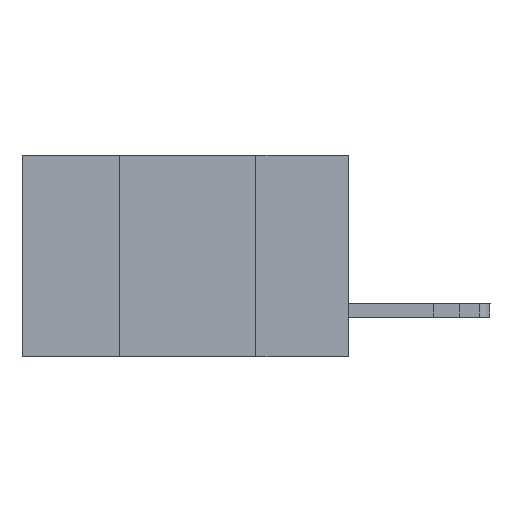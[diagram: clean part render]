
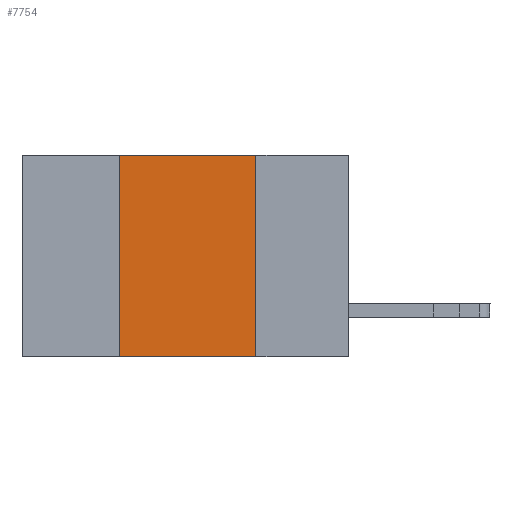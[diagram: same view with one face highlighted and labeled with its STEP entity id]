
A CAD part, left-side view. The second image highlights one B-rep face of the part: STEP entity #7754.
In plain terms, the highlighted planar face has unit normal (-1, 0, 0).
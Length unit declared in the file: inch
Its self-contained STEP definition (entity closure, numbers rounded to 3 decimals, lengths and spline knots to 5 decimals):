
#134 = ORIENTED_EDGE ( 'NONE', *, *, #7679, .F. ) ;
#285 = CARTESIAN_POINT ( 'NONE',  ( 0., 0.6, -0.37 ) ) ;
#486 = VECTOR ( 'NONE', #734, 39.37008 ) ;
#564 = CARTESIAN_POINT ( 'NONE',  ( 0., 0.42, 0. ) ) ;
#578 = VERTEX_POINT ( 'NONE', #10314 ) ;
#629 = CARTESIAN_POINT ( 'NONE',  ( 0., 0.42, -0.37 ) ) ;
#669 = CARTESIAN_POINT ( 'NONE',  ( 0., 0.6, 0. ) ) ;
#734 = DIRECTION ( 'NONE',  ( 0., 0., 1. ) ) ;
#1338 = DIRECTION ( 'NONE',  ( 0., -1., 0. ) ) ;
#1389 = VECTOR ( 'NONE', #5012, 39.37008 ) ;
#1519 = LINE ( 'NONE', #564, #486 ) ;
#1689 = EDGE_CURVE ( 'NONE', #7412, #578, #9276, .T. ) ;
#1795 = DIRECTION ( 'NONE',  ( 1., 0., 0. ) ) ;
#2260 = EDGE_LOOP ( 'NONE', ( #8542, #10179, #134, #9044 ) ) ;
#2490 = VERTEX_POINT ( 'NONE', #629 ) ;
#2897 = DIRECTION ( 'NONE',  ( 0., 0., -1. ) ) ;
#3389 = VECTOR ( 'NONE', #2897, 39.37008 ) ;
#3930 = VECTOR ( 'NONE', #1338, 39.37008 ) ;
#4408 = DIRECTION ( 'NONE',  ( 0., 0., -1. ) ) ;
#5012 = DIRECTION ( 'NONE',  ( 0., -1., 0. ) ) ;
#7232 = CARTESIAN_POINT ( 'NONE',  ( 0., 0.17, 0. ) ) ;
#7412 = VERTEX_POINT ( 'NONE', #10342 ) ;
#7679 = EDGE_CURVE ( 'NONE', #2490, #7412, #1519, .T. ) ;
#7754 = ADVANCED_FACE ( 'NONE', ( #9344 ), #8678, .F. ) ;
#8469 = VERTEX_POINT ( 'NONE', #9132 ) ;
#8542 = ORIENTED_EDGE ( 'NONE', *, *, #9476, .F. ) ;
#8678 = PLANE ( 'NONE',  #9589 ) ;
#9044 = ORIENTED_EDGE ( 'NONE', *, *, #9055, .T. ) ;
#9055 = EDGE_CURVE ( 'NONE', #2490, #8469, #10663, .T. ) ;
#9132 = CARTESIAN_POINT ( 'NONE',  ( 0., 0.17, -0.37 ) ) ;
#9276 = LINE ( 'NONE', #669, #1389 ) ;
#9344 = FACE_OUTER_BOUND ( 'NONE', #2260, .T. ) ;
#9397 = CARTESIAN_POINT ( 'NONE',  ( 0., 0.6, 0. ) ) ;
#9476 = EDGE_CURVE ( 'NONE', #578, #8469, #9601, .T. ) ;
#9589 = AXIS2_PLACEMENT_3D ( 'NONE', #9397, #1795, #4408 ) ;
#9601 = LINE ( 'NONE', #7232, #3389 ) ;
#10179 = ORIENTED_EDGE ( 'NONE', *, *, #1689, .F. ) ;
#10314 = CARTESIAN_POINT ( 'NONE',  ( 0., 0.17, 0. ) ) ;
#10342 = CARTESIAN_POINT ( 'NONE',  ( 0., 0.42, 0. ) ) ;
#10663 = LINE ( 'NONE', #285, #3930 ) ;
